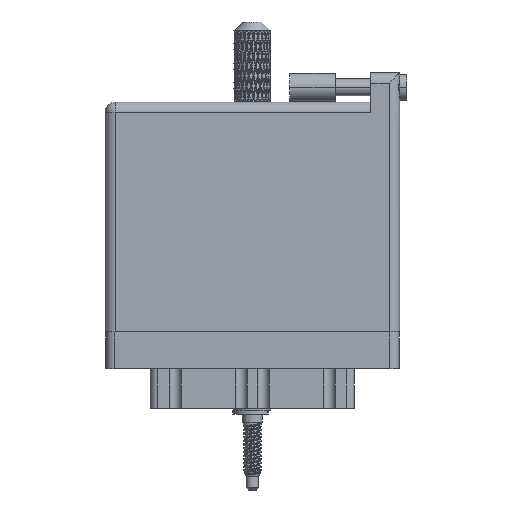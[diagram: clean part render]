
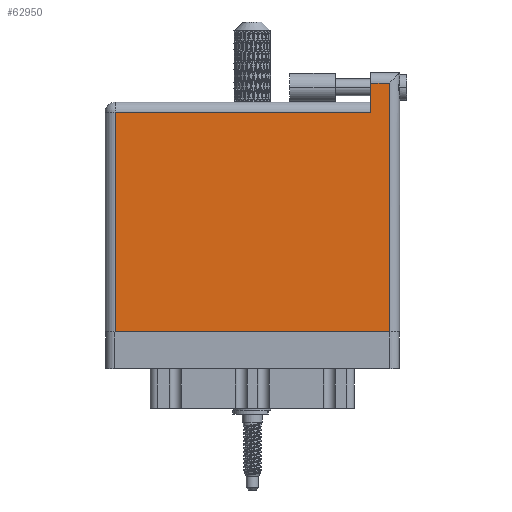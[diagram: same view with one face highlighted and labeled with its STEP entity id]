
A CAD part, front view. The second image highlights one B-rep face of the part: STEP entity #62950.
In plain terms, the highlighted face is planar.
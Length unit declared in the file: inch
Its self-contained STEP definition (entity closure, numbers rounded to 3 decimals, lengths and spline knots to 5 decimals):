
#723 = VECTOR ( 'NONE', #75079, 39.37008 ) ;
#4074 = DIRECTION ( 'NONE',  ( -1., 0., 0. ) ) ;
#5124 = EDGE_CURVE ( 'NONE', #63224, #41421, #96321, .T. ) ;
#6954 = AXIS2_PLACEMENT_3D ( 'NONE', #11683, #42646, #4074 ) ;
#7901 = LINE ( 'NONE', #9892, #88884 ) ;
#8539 = VERTEX_POINT ( 'NONE', #36567 ) ;
#9892 = CARTESIAN_POINT ( 'NONE',  ( 1.938, 1.766, 0. ) ) ;
#11683 = CARTESIAN_POINT ( 'NONE',  ( 0., 1.566, 0. ) ) ;
#13213 = VECTOR ( 'NONE', #57693, 39.37008 ) ;
#17009 = ORIENTED_EDGE ( 'NONE', *, *, #20241, .T. ) ;
#20241 = EDGE_CURVE ( 'NONE', #8539, #99074, #7901, .T. ) ;
#20723 = CARTESIAN_POINT ( 'NONE',  ( 0., 0., 0. ) ) ;
#20864 = LINE ( 'NONE', #43243, #40925 ) ;
#23929 = EDGE_CURVE ( 'NONE', #41421, #28624, #91521, .T. ) ;
#26164 = CARTESIAN_POINT ( 'NONE',  ( 1.811, 1.496, 0. ) ) ;
#26703 = CARTESIAN_POINT ( 'NONE',  ( 1.811, 1.766, 0. ) ) ;
#27284 = CARTESIAN_POINT ( 'NONE',  ( 1.811, 1.696, 0. ) ) ;
#28624 = VERTEX_POINT ( 'NONE', #79469 ) ;
#29060 = CARTESIAN_POINT ( 'NONE',  ( 0.07, 0., 0. ) ) ;
#36567 = CARTESIAN_POINT ( 'NONE',  ( 1.938, 0., 0. ) ) ;
#36784 = CARTESIAN_POINT ( 'NONE',  ( 1.938, 1.696, 0. ) ) ;
#37122 = CARTESIAN_POINT ( 'NONE',  ( 0.07, 0., 0. ) ) ;
#37454 = EDGE_CURVE ( 'NONE', #28624, #57481, #83926, .T. ) ;
#40925 = VECTOR ( 'NONE', #73221, 39.37008 ) ;
#41421 = VERTEX_POINT ( 'NONE', #26164 ) ;
#42646 = DIRECTION ( 'NONE',  ( 0., 0., -1. ) ) ;
#43243 = CARTESIAN_POINT ( 'NONE',  ( 0., 1.696, 0. ) ) ;
#44082 = LINE ( 'NONE', #20723, #723 ) ;
#44754 = DIRECTION ( 'NONE',  ( -1., 0., 0. ) ) ;
#50074 = VECTOR ( 'NONE', #71070, 39.37008 ) ;
#52269 = ORIENTED_EDGE ( 'NONE', *, *, #69012, .T. ) ;
#57481 = VERTEX_POINT ( 'NONE', #37122 ) ;
#57693 = DIRECTION ( 'NONE',  ( 0., -1., 0. ) ) ;
#59016 = ORIENTED_EDGE ( 'NONE', *, *, #23929, .T. ) ;
#61601 = EDGE_LOOP ( 'NONE', ( #52269, #17009, #90359, #87438, #59016, #77004 ) ) ;
#62950 = ADVANCED_FACE ( 'NONE', ( #74118 ), #81260, .F. ) ;
#63224 = VERTEX_POINT ( 'NONE', #27284 ) ;
#69012 = EDGE_CURVE ( 'NONE', #57481, #8539, #44082, .T. ) ;
#71070 = DIRECTION ( 'NONE',  ( 0., -1., 0. ) ) ;
#71880 = DIRECTION ( 'NONE',  ( 0., 1., 0. ) ) ;
#73221 = DIRECTION ( 'NONE',  ( -1., 0., 0. ) ) ;
#74118 = FACE_OUTER_BOUND ( 'NONE', #61601, .T. ) ;
#75079 = DIRECTION ( 'NONE',  ( 1., 0., 0. ) ) ;
#77004 = ORIENTED_EDGE ( 'NONE', *, *, #37454, .T. ) ;
#79469 = CARTESIAN_POINT ( 'NONE',  ( 0.07, 1.496, 0. ) ) ;
#81260 = PLANE ( 'NONE',  #6954 ) ;
#83524 = VECTOR ( 'NONE', #44754, 39.37008 ) ;
#83926 = LINE ( 'NONE', #29060, #50074 ) ;
#87438 = ORIENTED_EDGE ( 'NONE', *, *, #5124, .T. ) ;
#88884 = VECTOR ( 'NONE', #71880, 39.37008 ) ;
#90359 = ORIENTED_EDGE ( 'NONE', *, *, #98208, .T. ) ;
#91521 = LINE ( 'NONE', #98126, #83524 ) ;
#96321 = LINE ( 'NONE', #26703, #13213 ) ;
#98126 = CARTESIAN_POINT ( 'NONE',  ( 0., 1.496, 0. ) ) ;
#98208 = EDGE_CURVE ( 'NONE', #99074, #63224, #20864, .T. ) ;
#99074 = VERTEX_POINT ( 'NONE', #36784 ) ;
